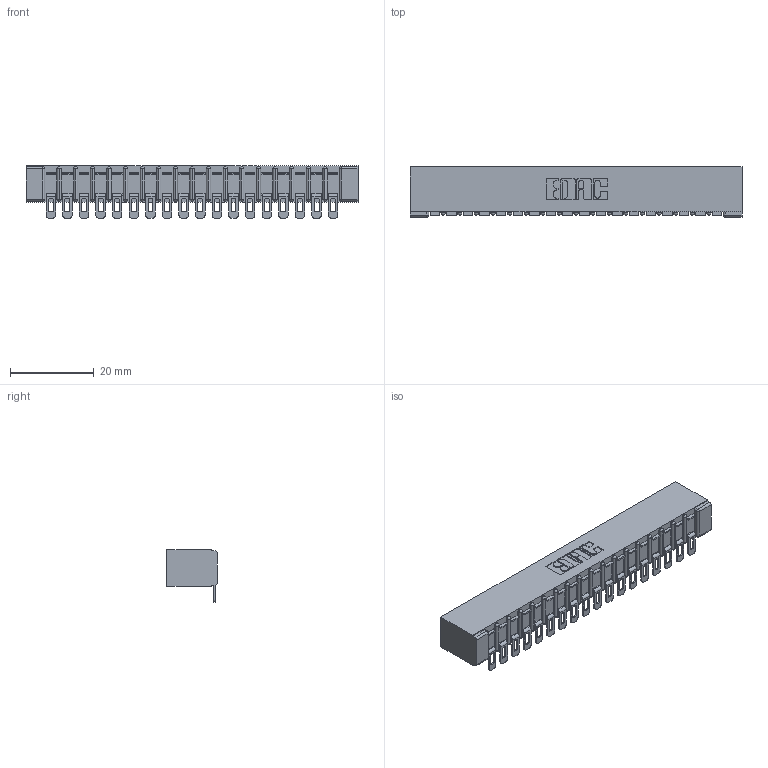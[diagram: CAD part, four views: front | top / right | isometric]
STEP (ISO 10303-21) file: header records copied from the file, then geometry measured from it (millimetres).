
FILE_DESCRIPTION (( 'STEP AP203' ), '1' );
FILE_NAME ('307-018-454-101.STEP', '2020-09-26T00:47:38', ( '' ), ( '' ), 'SwSTEP 2.0', 'SolidWorks 2020', '' );
FILE_SCHEMA (( 'CONFIG_CONTROL_DESIGN' ));
Length unit declared in the file: inch
Products named in the file (3): 307-290-002_554; 307 Part_No Mounting Lugs; 307-018-454-101
Assembly tree (19 placements, depth 2):
  307-018-454-101
    307 Part_No Mounting Lugs
    307-290-002_554  x18
Bounding box: 79.2 x 12.01 x 12.52 mm (x, y, z)
Volume: 5475.1 mm3; surface area: 10317.2 mm2
Topology: 19 solids, 19 shells, 1587 faces, 4853 edges, 3182 vertices
Faces by surface type: plane 894, cylinder 655, sphere 38
Entity records: 19077 total; most frequent: CARTESIAN_POINT 3214, ORIENTED_EDGE 3204, DIRECTION 3138, EDGE_CURVE 1602, VECTOR 1210, LINE 1210, VERTEX_POINT 1040, AXIS2_PLACEMENT_3D 964
